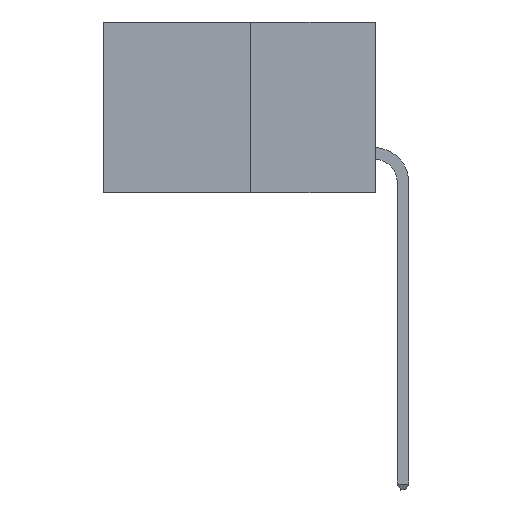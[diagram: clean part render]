
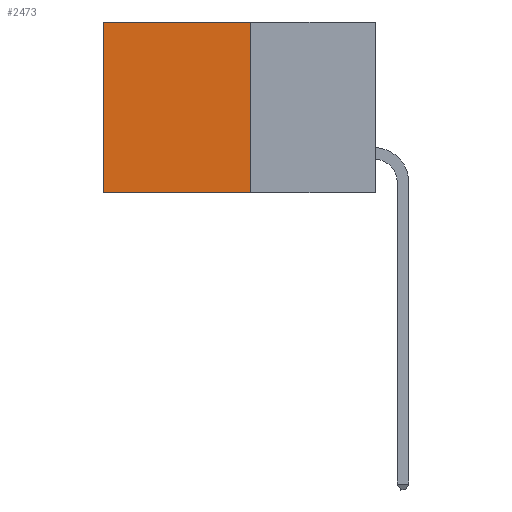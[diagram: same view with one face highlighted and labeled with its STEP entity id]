
A CAD part, left-side view. The second image highlights one B-rep face of the part: STEP entity #2473.
In plain terms, the highlighted planar face has unit normal (-1, 0, 0).
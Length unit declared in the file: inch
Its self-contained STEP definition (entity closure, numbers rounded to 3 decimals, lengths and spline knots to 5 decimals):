
#1158 = VERTEX_POINT ( 'NONE', #12849 ) ;
#1743 = LINE ( 'NONE', #9763, #7766 ) ;
#2258 = LINE ( 'NONE', #5946, #14355 ) ;
#2365 = CARTESIAN_POINT ( 'NONE',  ( 0.277, 0.59, -0.37 ) ) ;
#2409 = ORIENTED_EDGE ( 'NONE', *, *, #9379, .F. ) ;
#2473 = ADVANCED_FACE ( 'NONE', ( #13958 ), #2653, .F. ) ;
#2653 = PLANE ( 'NONE',  #11827 ) ;
#3869 = DIRECTION ( 'NONE',  ( 0., 1., 0. ) ) ;
#3894 = DIRECTION ( 'NONE',  ( 1., 0., 0. ) ) ;
#4185 = VERTEX_POINT ( 'NONE', #9431 ) ;
#4207 = CARTESIAN_POINT ( 'NONE',  ( 0.277, 0.59, -0.37 ) ) ;
#4358 = CARTESIAN_POINT ( 'NONE',  ( 0.277, 0.27, 0. ) ) ;
#4883 = LINE ( 'NONE', #4358, #7678 ) ;
#5946 = CARTESIAN_POINT ( 'NONE',  ( 0.277, 0.27, -0.37 ) ) ;
#6257 = VERTEX_POINT ( 'NONE', #7679 ) ;
#7678 = VECTOR ( 'NONE', #13666, 39.37008 ) ;
#7679 = CARTESIAN_POINT ( 'NONE',  ( 0.277, 0.27, -0.37 ) ) ;
#7766 = VECTOR ( 'NONE', #3869, 39.37008 ) ;
#7966 = EDGE_CURVE ( 'NONE', #6257, #9770, #1743, .T. ) ;
#8398 = ORIENTED_EDGE ( 'NONE', *, *, #7966, .F. ) ;
#8761 = EDGE_CURVE ( 'NONE', #1158, #9770, #14187, .T. ) ;
#9379 = EDGE_CURVE ( 'NONE', #4185, #6257, #2258, .T. ) ;
#9431 = CARTESIAN_POINT ( 'NONE',  ( 0.277, 0.27, 0. ) ) ;
#9763 = CARTESIAN_POINT ( 'NONE',  ( 0.277, 0.27, -0.37 ) ) ;
#9770 = VERTEX_POINT ( 'NONE', #4207 ) ;
#10543 = EDGE_CURVE ( 'NONE', #4185, #1158, #4883, .T. ) ;
#10685 = DIRECTION ( 'NONE',  ( 0., 0., -1. ) ) ;
#10686 = EDGE_LOOP ( 'NONE', ( #14129, #8398, #2409, #11840 ) ) ;
#10963 = CARTESIAN_POINT ( 'NONE',  ( 0.277, 0.27, -0.37 ) ) ;
#11827 = AXIS2_PLACEMENT_3D ( 'NONE', #10963, #3894, #12112 ) ;
#11840 = ORIENTED_EDGE ( 'NONE', *, *, #10543, .T. ) ;
#11906 = VECTOR ( 'NONE', #10685, 39.37008 ) ;
#12112 = DIRECTION ( 'NONE',  ( 0., 0., -1. ) ) ;
#12849 = CARTESIAN_POINT ( 'NONE',  ( 0.277, 0.59, 0. ) ) ;
#13666 = DIRECTION ( 'NONE',  ( 0., 1., 0. ) ) ;
#13958 = FACE_OUTER_BOUND ( 'NONE', #10686, .T. ) ;
#14129 = ORIENTED_EDGE ( 'NONE', *, *, #8761, .T. ) ;
#14187 = LINE ( 'NONE', #2365, #11906 ) ;
#14355 = VECTOR ( 'NONE', #15168, 39.37008 ) ;
#15168 = DIRECTION ( 'NONE',  ( 0., 0., -1. ) ) ;
